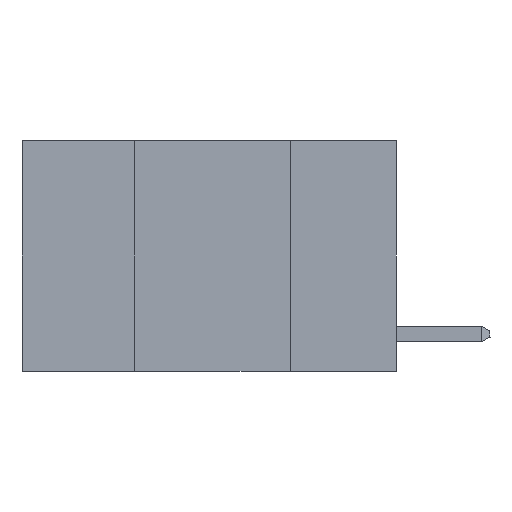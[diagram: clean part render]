
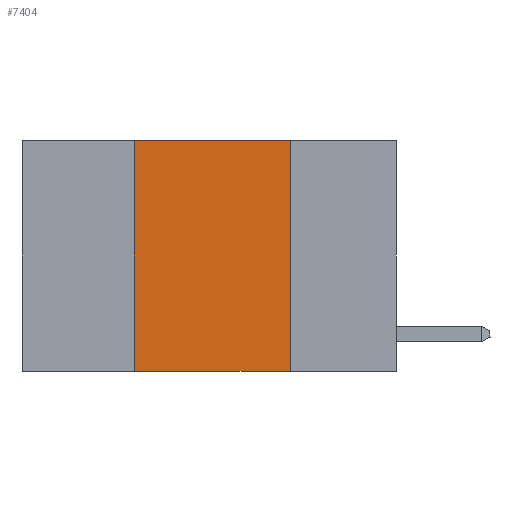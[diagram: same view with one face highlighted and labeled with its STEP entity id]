
A CAD part, left-side view. The second image highlights one B-rep face of the part: STEP entity #7404.
In plain terms, the highlighted planar face has unit normal (-1, 0, 0).
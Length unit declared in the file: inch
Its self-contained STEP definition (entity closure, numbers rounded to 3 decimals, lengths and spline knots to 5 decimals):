
#764 = VERTEX_POINT ( 'NONE', #10516 ) ;
#1069 = VERTEX_POINT ( 'NONE', #3334 ) ;
#1250 = LINE ( 'NONE', #6824, #3503 ) ;
#1724 = DIRECTION ( 'NONE',  ( 0., -1., 0. ) ) ;
#1898 = ORIENTED_EDGE ( 'NONE', *, *, #7200, .F. ) ;
#1926 = AXIS2_PLACEMENT_3D ( 'NONE', #1985, #2840, #8806 ) ;
#1985 = CARTESIAN_POINT ( 'NONE',  ( 0., 0.6, 0. ) ) ;
#2129 = LINE ( 'NONE', #4682, #4405 ) ;
#2419 = EDGE_LOOP ( 'NONE', ( #6169, #10600, #1898, #6436 ) ) ;
#2546 = VECTOR ( 'NONE', #7830, 39.37008 ) ;
#2711 = CARTESIAN_POINT ( 'NONE',  ( 0., 0.17, 0. ) ) ;
#2803 = LINE ( 'NONE', #2711, #2546 ) ;
#2840 = DIRECTION ( 'NONE',  ( 1., 0., 0. ) ) ;
#3334 = CARTESIAN_POINT ( 'NONE',  ( 0., 0.42, 0. ) ) ;
#3503 = VECTOR ( 'NONE', #1724, 39.37008 ) ;
#3777 = VECTOR ( 'NONE', #10154, 39.37008 ) ;
#4364 = VERTEX_POINT ( 'NONE', #7549 ) ;
#4405 = VECTOR ( 'NONE', #8918, 39.37008 ) ;
#4682 = CARTESIAN_POINT ( 'NONE',  ( 0., 0.6, -0.37 ) ) ;
#4801 = VERTEX_POINT ( 'NONE', #6482 ) ;
#5142 = CARTESIAN_POINT ( 'NONE',  ( 0., 0.42, 0. ) ) ;
#5906 = FACE_OUTER_BOUND ( 'NONE', #2419, .T. ) ;
#6169 = ORIENTED_EDGE ( 'NONE', *, *, #8474, .F. ) ;
#6436 = ORIENTED_EDGE ( 'NONE', *, *, #9186, .T. ) ;
#6482 = CARTESIAN_POINT ( 'NONE',  ( 0., 0.17, 0. ) ) ;
#6500 = EDGE_CURVE ( 'NONE', #1069, #4801, #1250, .T. ) ;
#6824 = CARTESIAN_POINT ( 'NONE',  ( 0., 0.6, 0. ) ) ;
#7104 = PLANE ( 'NONE',  #1926 ) ;
#7200 = EDGE_CURVE ( 'NONE', #4364, #1069, #10230, .T. ) ;
#7404 = ADVANCED_FACE ( 'NONE', ( #5906 ), #7104, .F. ) ;
#7549 = CARTESIAN_POINT ( 'NONE',  ( 0., 0.42, -0.37 ) ) ;
#7830 = DIRECTION ( 'NONE',  ( 0., 0., -1. ) ) ;
#8474 = EDGE_CURVE ( 'NONE', #4801, #764, #2803, .T. ) ;
#8806 = DIRECTION ( 'NONE',  ( 0., 0., -1. ) ) ;
#8918 = DIRECTION ( 'NONE',  ( 0., -1., 0. ) ) ;
#9186 = EDGE_CURVE ( 'NONE', #4364, #764, #2129, .T. ) ;
#10154 = DIRECTION ( 'NONE',  ( 0., 0., 1. ) ) ;
#10230 = LINE ( 'NONE', #5142, #3777 ) ;
#10516 = CARTESIAN_POINT ( 'NONE',  ( 0., 0.17, -0.37 ) ) ;
#10600 = ORIENTED_EDGE ( 'NONE', *, *, #6500, .F. ) ;
